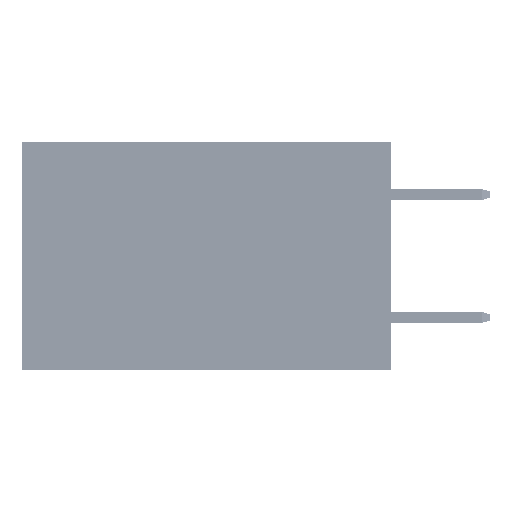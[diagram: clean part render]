
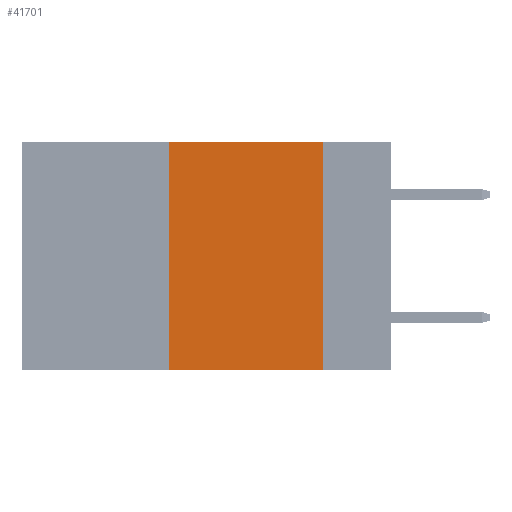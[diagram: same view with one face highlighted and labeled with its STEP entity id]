
A CAD part, left-side view. The second image highlights one B-rep face of the part: STEP entity #41701.
In plain terms, the highlighted planar face has unit normal (-1, 0, 0).
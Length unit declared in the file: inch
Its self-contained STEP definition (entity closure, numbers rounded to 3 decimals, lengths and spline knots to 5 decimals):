
#565 = EDGE_CURVE ( 'NONE', #27071, #41346, #43193, .T. ) ;
#725 = CARTESIAN_POINT ( 'NONE',  ( 0., 0.6, 0. ) ) ;
#8673 = DIRECTION ( 'NONE',  ( 1., 0., 0. ) ) ;
#9375 = EDGE_CURVE ( 'NONE', #41346, #30365, #43825, .T. ) ;
#9600 = ORIENTED_EDGE ( 'NONE', *, *, #28157, .T. ) ;
#11052 = CARTESIAN_POINT ( 'NONE',  ( 0., 0.36, -0.37 ) ) ;
#11723 = EDGE_LOOP ( 'NONE', ( #23262, #32052, #35449, #9600 ) ) ;
#12537 = DIRECTION ( 'NONE',  ( 0., -1., 0. ) ) ;
#13768 = CARTESIAN_POINT ( 'NONE',  ( 0., 0.11, 0. ) ) ;
#15764 = DIRECTION ( 'NONE',  ( 0., -1., 0. ) ) ;
#16031 = LINE ( 'NONE', #20014, #27011 ) ;
#16369 = AXIS2_PLACEMENT_3D ( 'NONE', #725, #8673, #33648 ) ;
#17146 = CARTESIAN_POINT ( 'NONE',  ( 0., 0.11, -0.37 ) ) ;
#18298 = CARTESIAN_POINT ( 'NONE',  ( 0., 0.36, 0. ) ) ;
#20014 = CARTESIAN_POINT ( 'NONE',  ( 0., 0.6, -0.37 ) ) ;
#23008 = CARTESIAN_POINT ( 'NONE',  ( 0., 0.6, 0. ) ) ;
#23262 = ORIENTED_EDGE ( 'NONE', *, *, #9375, .F. ) ;
#25656 = CARTESIAN_POINT ( 'NONE',  ( 0., 0.36, 0. ) ) ;
#27011 = VECTOR ( 'NONE', #15764, 39.37008 ) ;
#27071 = VERTEX_POINT ( 'NONE', #18298 ) ;
#28157 = EDGE_CURVE ( 'NONE', #31891, #30365, #16031, .T. ) ;
#30365 = VERTEX_POINT ( 'NONE', #17146 ) ;
#31891 = VERTEX_POINT ( 'NONE', #11052 ) ;
#32052 = ORIENTED_EDGE ( 'NONE', *, *, #565, .F. ) ;
#33648 = DIRECTION ( 'NONE',  ( 0., 0., -1. ) ) ;
#34304 = VECTOR ( 'NONE', #12537, 39.37008 ) ;
#35449 = ORIENTED_EDGE ( 'NONE', *, *, #48693, .F. ) ;
#37113 = FACE_OUTER_BOUND ( 'NONE', #11723, .T. ) ;
#40431 = VECTOR ( 'NONE', #47548, 39.37008 ) ;
#41346 = VERTEX_POINT ( 'NONE', #13768 ) ;
#41701 = ADVANCED_FACE ( 'NONE', ( #37113 ), #45076, .F. ) ;
#43193 = LINE ( 'NONE', #23008, #34304 ) ;
#43825 = LINE ( 'NONE', #51779, #40431 ) ;
#45076 = PLANE ( 'NONE',  #16369 ) ;
#45841 = LINE ( 'NONE', #25656, #51994 ) ;
#46090 = DIRECTION ( 'NONE',  ( 0., 0., 1. ) ) ;
#47548 = DIRECTION ( 'NONE',  ( 0., 0., -1. ) ) ;
#48693 = EDGE_CURVE ( 'NONE', #31891, #27071, #45841, .T. ) ;
#51779 = CARTESIAN_POINT ( 'NONE',  ( 0., 0.11, 0. ) ) ;
#51994 = VECTOR ( 'NONE', #46090, 39.37008 ) ;
